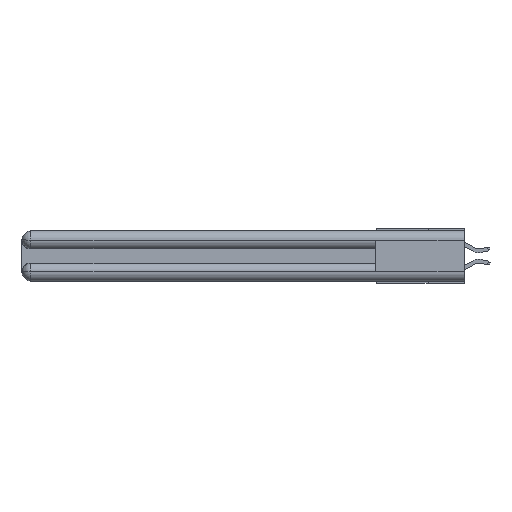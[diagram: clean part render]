
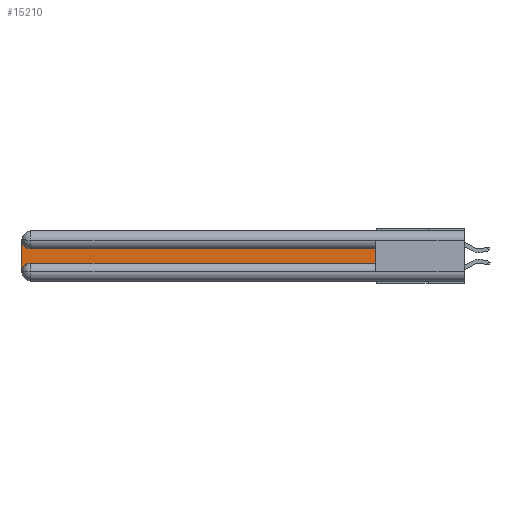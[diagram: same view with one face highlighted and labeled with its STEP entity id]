
A CAD part, left-side view. The second image highlights one B-rep face of the part: STEP entity #15210.
In plain terms, the highlighted planar face has unit normal (-1, 0, 0).
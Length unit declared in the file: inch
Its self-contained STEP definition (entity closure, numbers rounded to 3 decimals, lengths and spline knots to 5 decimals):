
#169 = VERTEX_POINT ( 'NONE', #11127 ) ;
#412 = VERTEX_POINT ( 'NONE', #6738 ) ;
#1664 = VECTOR ( 'NONE', #7981, 39.37008 ) ;
#1751 = VECTOR ( 'NONE', #2494, 39.37008 ) ;
#2494 = DIRECTION ( 'NONE',  ( 0., -1., 0. ) ) ;
#3077 = CIRCLE ( 'NONE', #27499, 0.06 ) ;
#3116 = CARTESIAN_POINT ( 'NONE',  ( 0.075, 3., -0.2175 ) ) ;
#3320 = LINE ( 'NONE', #13061, #24273 ) ;
#3366 = ORIENTED_EDGE ( 'NONE', *, *, #8191, .T. ) ;
#4072 = VERTEX_POINT ( 'NONE', #6045 ) ;
#5783 = DIRECTION ( 'NONE',  ( 0., 0., 1. ) ) ;
#5814 = ORIENTED_EDGE ( 'NONE', *, *, #16332, .T. ) ;
#6045 = CARTESIAN_POINT ( 'NONE',  ( 0.075, 3., -0.0625 ) ) ;
#6423 = EDGE_CURVE ( 'NONE', #29735, #4072, #3077, .T. ) ;
#6738 = CARTESIAN_POINT ( 'NONE',  ( 0.075, 2.94, -0.2175 ) ) ;
#6927 = ORIENTED_EDGE ( 'NONE', *, *, #15737, .T. ) ;
#7981 = DIRECTION ( 'NONE',  ( 0., 0., -1. ) ) ;
#8191 = EDGE_CURVE ( 'NONE', #169, #412, #22306, .T. ) ;
#9617 = LINE ( 'NONE', #30431, #18074 ) ;
#9690 = CARTESIAN_POINT ( 'NONE',  ( 0.075, 0.6, -0.2175 ) ) ;
#11127 = CARTESIAN_POINT ( 'NONE',  ( 0.075, 3., -0.2775 ) ) ;
#11519 = AXIS2_PLACEMENT_3D ( 'NONE', #15647, #27766, #17753 ) ;
#12877 = CARTESIAN_POINT ( 'NONE',  ( 0.075, 2.94, -0.1225 ) ) ;
#13061 = CARTESIAN_POINT ( 'NONE',  ( 0.075, 0.6, -0.2175 ) ) ;
#13775 = CARTESIAN_POINT ( 'NONE',  ( 0.075, 2.94, -0.0625 ) ) ;
#15040 = DIRECTION ( 'NONE',  ( 0., 0., -1. ) ) ;
#15102 = EDGE_LOOP ( 'NONE', ( #25304, #16000, #27948, #3366, #5814, #6927 ) ) ;
#15210 = ADVANCED_FACE ( 'NONE', ( #17805 ), #20413, .F. ) ;
#15647 = CARTESIAN_POINT ( 'NONE',  ( 0.075, 3., -0.1225 ) ) ;
#15737 = EDGE_CURVE ( 'NONE', #19419, #25567, #3320, .T. ) ;
#16000 = ORIENTED_EDGE ( 'NONE', *, *, #6423, .T. ) ;
#16222 = DIRECTION ( 'NONE',  ( 1., 0., 0. ) ) ;
#16332 = EDGE_CURVE ( 'NONE', #412, #19419, #20445, .T. ) ;
#17620 = EDGE_CURVE ( 'NONE', #4072, #169, #19959, .T. ) ;
#17753 = DIRECTION ( 'NONE',  ( 0., 0., -1. ) ) ;
#17805 = FACE_OUTER_BOUND ( 'NONE', #15102, .T. ) ;
#18074 = VECTOR ( 'NONE', #23163, 39.37008 ) ;
#18666 = DIRECTION ( 'NONE',  ( 0., 0., -1. ) ) ;
#19419 = VERTEX_POINT ( 'NONE', #20331 ) ;
#19959 = LINE ( 'NONE', #3116, #1664 ) ;
#20331 = CARTESIAN_POINT ( 'NONE',  ( 0.075, 0.6, -0.2175 ) ) ;
#20413 = PLANE ( 'NONE',  #11519 ) ;
#20445 = LINE ( 'NONE', #9690, #1751 ) ;
#22306 = CIRCLE ( 'NONE', #29610, 0.06 ) ;
#23163 = DIRECTION ( 'NONE',  ( 0., 1., 0. ) ) ;
#24165 = CARTESIAN_POINT ( 'NONE',  ( 0.075, 2.94, -0.2775 ) ) ;
#24273 = VECTOR ( 'NONE', #5783, 39.37008 ) ;
#24988 = CARTESIAN_POINT ( 'NONE',  ( 0.075, 0.6, -0.1225 ) ) ;
#25304 = ORIENTED_EDGE ( 'NONE', *, *, #26875, .T. ) ;
#25567 = VERTEX_POINT ( 'NONE', #24988 ) ;
#26875 = EDGE_CURVE ( 'NONE', #25567, #29735, #9617, .T. ) ;
#27179 = DIRECTION ( 'NONE',  ( 1., 0., 0. ) ) ;
#27499 = AXIS2_PLACEMENT_3D ( 'NONE', #13775, #16222, #18666 ) ;
#27766 = DIRECTION ( 'NONE',  ( 1., 0., 0. ) ) ;
#27948 = ORIENTED_EDGE ( 'NONE', *, *, #17620, .T. ) ;
#29610 = AXIS2_PLACEMENT_3D ( 'NONE', #24165, #27179, #15040 ) ;
#29735 = VERTEX_POINT ( 'NONE', #12877 ) ;
#30431 = CARTESIAN_POINT ( 'NONE',  ( 0.075, 0.6, -0.1225 ) ) ;
